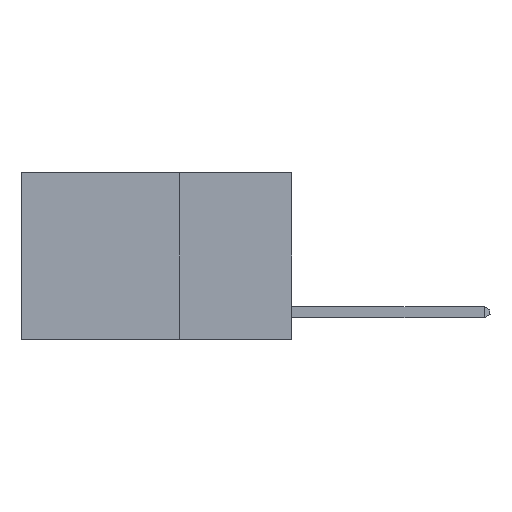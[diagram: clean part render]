
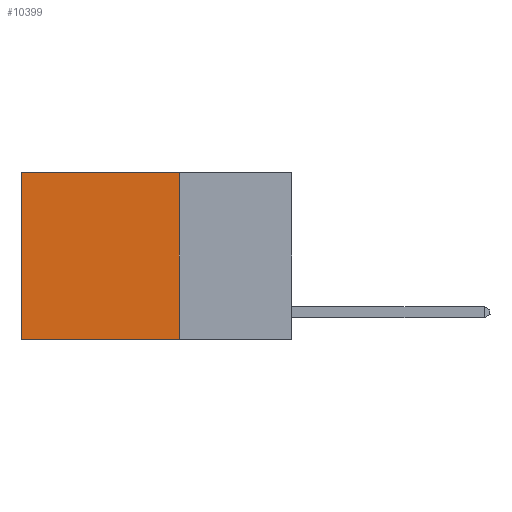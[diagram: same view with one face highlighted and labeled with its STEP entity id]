
A CAD part, left-side view. The second image highlights one B-rep face of the part: STEP entity #10399.
In plain terms, the highlighted planar face has unit normal (-1, 0, 0).
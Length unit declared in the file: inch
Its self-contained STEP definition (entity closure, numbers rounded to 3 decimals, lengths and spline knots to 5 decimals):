
#289 = VERTEX_POINT ( 'NONE', #10270 ) ;
#536 = ORIENTED_EDGE ( 'NONE', *, *, #9956, .F. ) ;
#577 = CARTESIAN_POINT ( 'NONE',  ( 0.2625, 0.6, 0. ) ) ;
#938 = DIRECTION ( 'NONE',  ( 1., 0., 0. ) ) ;
#1326 = LINE ( 'NONE', #9379, #11789 ) ;
#1478 = EDGE_CURVE ( 'NONE', #7414, #289, #1326, .T. ) ;
#1529 = VECTOR ( 'NONE', #10843, 39.37008 ) ;
#1587 = DIRECTION ( 'NONE',  ( 0., 0., -1. ) ) ;
#1822 = DIRECTION ( 'NONE',  ( 0., 0., -1. ) ) ;
#2565 = AXIS2_PLACEMENT_3D ( 'NONE', #10632, #938, #1822 ) ;
#3332 = DIRECTION ( 'NONE',  ( 0., 1., 0. ) ) ;
#3795 = ORIENTED_EDGE ( 'NONE', *, *, #7865, .T. ) ;
#5547 = VERTEX_POINT ( 'NONE', #12683 ) ;
#5869 = PLANE ( 'NONE',  #2565 ) ;
#6035 = DIRECTION ( 'NONE',  ( 0., 0., -1. ) ) ;
#6717 = FACE_OUTER_BOUND ( 'NONE', #6908, .T. ) ;
#6908 = EDGE_LOOP ( 'NONE', ( #9701, #536, #11688, #3795 ) ) ;
#7414 = VERTEX_POINT ( 'NONE', #577 ) ;
#7865 = EDGE_CURVE ( 'NONE', #9302, #7414, #8968, .T. ) ;
#7934 = CARTESIAN_POINT ( 'NONE',  ( 0.2625, 0.25, 0. ) ) ;
#8143 = VECTOR ( 'NONE', #6035, 39.37008 ) ;
#8144 = LINE ( 'NONE', #9055, #8143 ) ;
#8968 = LINE ( 'NONE', #7934, #12589 ) ;
#9055 = CARTESIAN_POINT ( 'NONE',  ( 0.2625, 0.25, 0. ) ) ;
#9216 = CARTESIAN_POINT ( 'NONE',  ( 0.2625, 0.25, 0. ) ) ;
#9302 = VERTEX_POINT ( 'NONE', #9216 ) ;
#9379 = CARTESIAN_POINT ( 'NONE',  ( 0.2625, 0.6, 0. ) ) ;
#9701 = ORIENTED_EDGE ( 'NONE', *, *, #1478, .T. ) ;
#9835 = CARTESIAN_POINT ( 'NONE',  ( 0.2625, 0.25, -0.37 ) ) ;
#9956 = EDGE_CURVE ( 'NONE', #5547, #289, #12443, .T. ) ;
#10270 = CARTESIAN_POINT ( 'NONE',  ( 0.2625, 0.6, -0.37 ) ) ;
#10399 = ADVANCED_FACE ( 'NONE', ( #6717 ), #5869, .F. ) ;
#10632 = CARTESIAN_POINT ( 'NONE',  ( 0.2625, 0.25, 0. ) ) ;
#10843 = DIRECTION ( 'NONE',  ( 0., 1., 0. ) ) ;
#11688 = ORIENTED_EDGE ( 'NONE', *, *, #12264, .F. ) ;
#11789 = VECTOR ( 'NONE', #1587, 39.37008 ) ;
#12264 = EDGE_CURVE ( 'NONE', #9302, #5547, #8144, .T. ) ;
#12443 = LINE ( 'NONE', #9835, #1529 ) ;
#12589 = VECTOR ( 'NONE', #3332, 39.37008 ) ;
#12683 = CARTESIAN_POINT ( 'NONE',  ( 0.2625, 0.25, -0.37 ) ) ;
